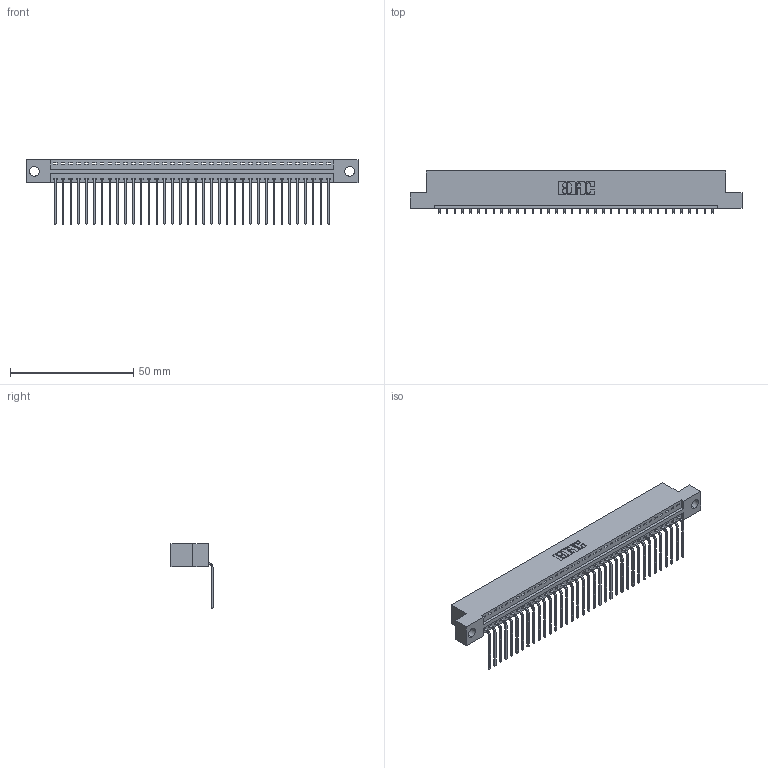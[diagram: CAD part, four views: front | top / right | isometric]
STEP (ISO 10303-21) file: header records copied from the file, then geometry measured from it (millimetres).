
FILE_DESCRIPTION (( 'STEP AP203' ), '1' );
FILE_NAME ('346-036-559-104.STEP', '2022-05-07T01:43:29', ( '' ), ( '' ), 'SwSTEP 2.0', 'SolidWorks 2020', '' );
FILE_SCHEMA (( 'CONFIG_CONTROL_DESIGN' ));
Length unit declared in the file: inch
Products named in the file (3): 346-036-559-104; 345-292-001_558 559 Tail - 1; 346 Part_Flush Mounting Lugs - 0.156 Dia-TH
Assembly tree (37 placements, depth 2):
  346-036-559-104
    346 Part_Flush Mounting Lugs - 0.156 Dia-TH
    345-292-001_558 559 Tail - 1  x36
Bounding box: 134.87 x 17.08 x 26.16 mm (x, y, z)
Volume: 12883.1 mm3; surface area: 16590.3 mm2
Topology: 37 solids, 37 shells, 2296 faces, 6917 edges, 4562 vertices
Faces by surface type: plane 1602, cylinder 694
Entity records: 23653 total; most frequent: CARTESIAN_POINT 4066, ORIENTED_EDGE 4034, DIRECTION 3593, EDGE_CURVE 2017, VECTOR 1741, LINE 1741, VERTEX_POINT 1342, AXIS2_PLACEMENT_3D 926
